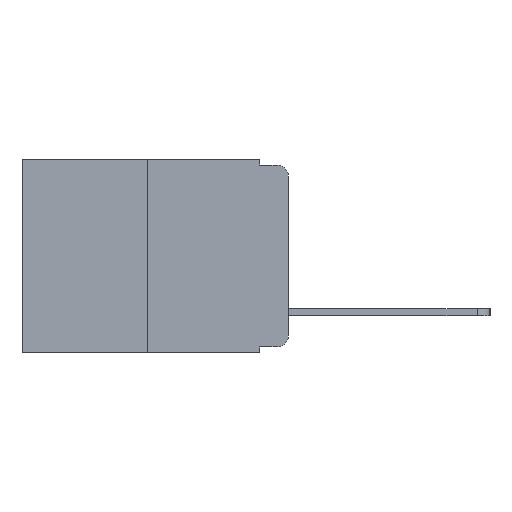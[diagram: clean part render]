
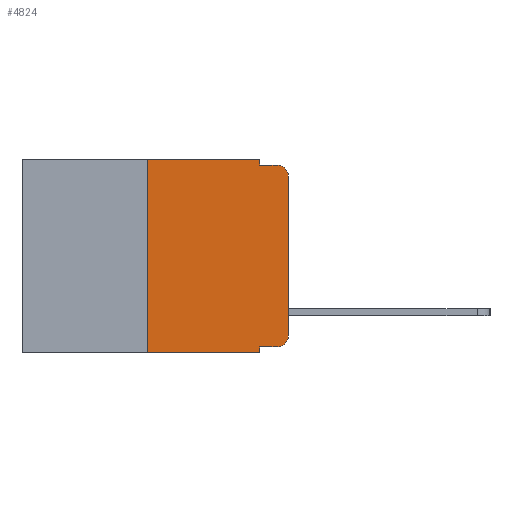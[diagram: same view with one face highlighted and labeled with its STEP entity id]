
A CAD part, left-side view. The second image highlights one B-rep face of the part: STEP entity #4824.
In plain terms, the highlighted planar face has unit normal (-1, 0, 0).
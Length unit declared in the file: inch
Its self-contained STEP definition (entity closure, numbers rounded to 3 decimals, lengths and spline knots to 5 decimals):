
#113 = FACE_OUTER_BOUND ( 'NONE', #516, .T. ) ;
#319 = CARTESIAN_POINT ( 'NONE',  ( 0., 0.051, -0.01 ) ) ;
#516 = EDGE_LOOP ( 'NONE', ( #9766, #7912, #8467, #6886, #6444, #6297, #11736, #2895, #8493, #4622 ) ) ;
#742 = DIRECTION ( 'NONE',  ( 1., 0., 0. ) ) ;
#1426 = CARTESIAN_POINT ( 'NONE',  ( 0., 0.02, -0.313 ) ) ;
#1536 = VERTEX_POINT ( 'NONE', #4616 ) ;
#1791 = VECTOR ( 'NONE', #7528, 39.37008 ) ;
#1968 = LINE ( 'NONE', #5707, #9681 ) ;
#2241 = CARTESIAN_POINT ( 'NONE',  ( 0., 0., -0.03 ) ) ;
#2297 = EDGE_CURVE ( 'NONE', #9164, #8416, #11513, .T. ) ;
#2345 = DIRECTION ( 'NONE',  ( 0., 0., 1. ) ) ;
#2403 = CARTESIAN_POINT ( 'NONE',  ( 0., 0., -0.313 ) ) ;
#2472 = DIRECTION ( 'NONE',  ( 0., 0., -1. ) ) ;
#2687 = CARTESIAN_POINT ( 'NONE',  ( 0., 0.02, -0.03 ) ) ;
#2895 = ORIENTED_EDGE ( 'NONE', *, *, #9662, .F. ) ;
#2938 = CARTESIAN_POINT ( 'NONE',  ( 0., 0.051, -0.01 ) ) ;
#3166 = DIRECTION ( 'NONE',  ( 0., 0., -1. ) ) ;
#3561 = CARTESIAN_POINT ( 'NONE',  ( 0., 0.051, -0.343 ) ) ;
#3721 = DIRECTION ( 'NONE',  ( 0., 0., -1. ) ) ;
#3955 = DIRECTION ( 'NONE',  ( 0., -1., 0. ) ) ;
#4209 = VERTEX_POINT ( 'NONE', #8379 ) ;
#4485 = LINE ( 'NONE', #6573, #1791 ) ;
#4588 = EDGE_CURVE ( 'NONE', #4209, #9618, #7649, .T. ) ;
#4616 = CARTESIAN_POINT ( 'NONE',  ( 0., 0.02, -0.01 ) ) ;
#4622 = ORIENTED_EDGE ( 'NONE', *, *, #4588, .T. ) ;
#4745 = EDGE_CURVE ( 'NONE', #11083, #1536, #8622, .T. ) ;
#4746 = AXIS2_PLACEMENT_3D ( 'NONE', #2687, #9428, #3721 ) ;
#4824 = ADVANCED_FACE ( 'NONE', ( #113 ), #11296, .F. ) ;
#5284 = VECTOR ( 'NONE', #9227, 39.37008 ) ;
#5631 = VERTEX_POINT ( 'NONE', #7450 ) ;
#5637 = VERTEX_POINT ( 'NONE', #3561 ) ;
#5666 = EDGE_CURVE ( 'NONE', #5631, #9164, #4485, .T. ) ;
#5707 = CARTESIAN_POINT ( 'NONE',  ( 0., 0., 0. ) ) ;
#5891 = EDGE_CURVE ( 'NONE', #9023, #4209, #12496, .T. ) ;
#5926 = LINE ( 'NONE', #2938, #10554 ) ;
#6297 = ORIENTED_EDGE ( 'NONE', *, *, #10241, .F. ) ;
#6397 = LINE ( 'NONE', #10998, #7006 ) ;
#6423 = CARTESIAN_POINT ( 'NONE',  ( 0., 0.051, -0.333 ) ) ;
#6444 = ORIENTED_EDGE ( 'NONE', *, *, #5666, .F. ) ;
#6573 = CARTESIAN_POINT ( 'NONE',  ( 0., 0.473, 0. ) ) ;
#6886 = ORIENTED_EDGE ( 'NONE', *, *, #2297, .F. ) ;
#6898 = CARTESIAN_POINT ( 'NONE',  ( 0., 0.25, -0.343 ) ) ;
#7006 = VECTOR ( 'NONE', #7416, 39.37008 ) ;
#7032 = CARTESIAN_POINT ( 'NONE',  ( 0., 0.051, 0. ) ) ;
#7416 = DIRECTION ( 'NONE',  ( 0., 0., -1. ) ) ;
#7450 = CARTESIAN_POINT ( 'NONE',  ( 0., 0.25, 0. ) ) ;
#7528 = DIRECTION ( 'NONE',  ( 0., -1., 0. ) ) ;
#7649 = CIRCLE ( 'NONE', #8803, 0.02 ) ;
#7706 = DIRECTION ( 'NONE',  ( 0., 0., -1. ) ) ;
#7912 = ORIENTED_EDGE ( 'NONE', *, *, #4745, .T. ) ;
#7974 = AXIS2_PLACEMENT_3D ( 'NONE', #9509, #742, #7706 ) ;
#8290 = CARTESIAN_POINT ( 'NONE',  ( 0., 0.473, -0.343 ) ) ;
#8297 = DIRECTION ( 'NONE',  ( -1., 0., 0. ) ) ;
#8379 = CARTESIAN_POINT ( 'NONE',  ( 0., 0.02, -0.333 ) ) ;
#8416 = VERTEX_POINT ( 'NONE', #319 ) ;
#8467 = ORIENTED_EDGE ( 'NONE', *, *, #10029, .F. ) ;
#8493 = ORIENTED_EDGE ( 'NONE', *, *, #5891, .T. ) ;
#8563 = VECTOR ( 'NONE', #2345, 39.37008 ) ;
#8622 = CIRCLE ( 'NONE', #4746, 0.02 ) ;
#8803 = AXIS2_PLACEMENT_3D ( 'NONE', #1426, #8297, #2472 ) ;
#8877 = CARTESIAN_POINT ( 'NONE',  ( 0., 0.051, -0.333 ) ) ;
#9023 = VERTEX_POINT ( 'NONE', #8877 ) ;
#9135 = VECTOR ( 'NONE', #3166, 39.37008 ) ;
#9164 = VERTEX_POINT ( 'NONE', #11403 ) ;
#9227 = DIRECTION ( 'NONE',  ( 0., -1., 0. ) ) ;
#9428 = DIRECTION ( 'NONE',  ( -1., 0., 0. ) ) ;
#9509 = CARTESIAN_POINT ( 'NONE',  ( 0., 0.473, 0. ) ) ;
#9618 = VERTEX_POINT ( 'NONE', #2403 ) ;
#9662 = EDGE_CURVE ( 'NONE', #9023, #5637, #6397, .T. ) ;
#9681 = VECTOR ( 'NONE', #12152, 39.37008 ) ;
#9766 = ORIENTED_EDGE ( 'NONE', *, *, #12217, .T. ) ;
#10029 = EDGE_CURVE ( 'NONE', #8416, #1536, #5926, .T. ) ;
#10127 = DIRECTION ( 'NONE',  ( 0., -1., 0. ) ) ;
#10241 = EDGE_CURVE ( 'NONE', #12380, #5631, #10962, .T. ) ;
#10554 = VECTOR ( 'NONE', #3955, 39.37008 ) ;
#10962 = LINE ( 'NONE', #11783, #8563 ) ;
#10998 = CARTESIAN_POINT ( 'NONE',  ( 0., 0.051, 0. ) ) ;
#11083 = VERTEX_POINT ( 'NONE', #2241 ) ;
#11269 = EDGE_CURVE ( 'NONE', #12380, #5637, #12088, .T. ) ;
#11296 = PLANE ( 'NONE',  #7974 ) ;
#11403 = CARTESIAN_POINT ( 'NONE',  ( 0., 0.051, 0. ) ) ;
#11513 = LINE ( 'NONE', #7032, #9135 ) ;
#11736 = ORIENTED_EDGE ( 'NONE', *, *, #11269, .T. ) ;
#11783 = CARTESIAN_POINT ( 'NONE',  ( 0., 0.25, 0. ) ) ;
#12088 = LINE ( 'NONE', #8290, #5284 ) ;
#12152 = DIRECTION ( 'NONE',  ( 0., 0., 1. ) ) ;
#12187 = VECTOR ( 'NONE', #10127, 39.37008 ) ;
#12217 = EDGE_CURVE ( 'NONE', #9618, #11083, #1968, .T. ) ;
#12380 = VERTEX_POINT ( 'NONE', #6898 ) ;
#12496 = LINE ( 'NONE', #6423, #12187 ) ;
